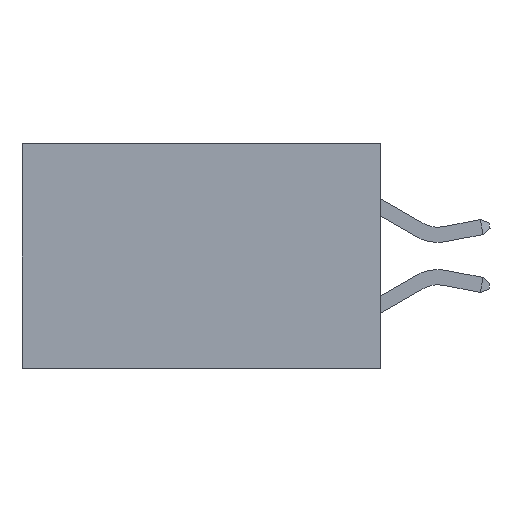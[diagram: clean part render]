
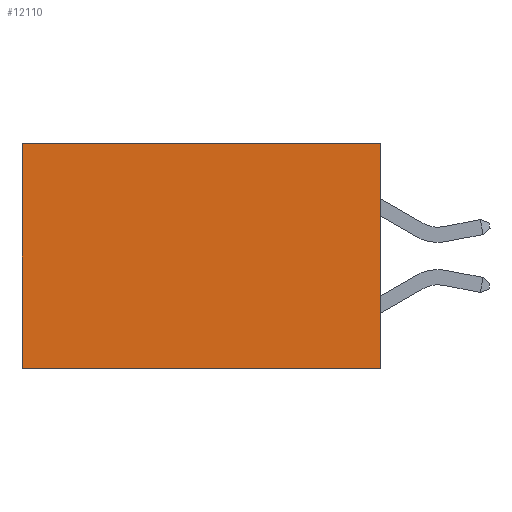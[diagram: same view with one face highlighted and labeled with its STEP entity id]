
A CAD part, left-side view. The second image highlights one B-rep face of the part: STEP entity #12110.
In plain terms, the highlighted planar face has unit normal (-1, 0, 0).
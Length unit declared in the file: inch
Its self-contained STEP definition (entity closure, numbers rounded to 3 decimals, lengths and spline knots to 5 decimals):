
#2889 = EDGE_CURVE ( 'NONE', #26231, #6369, #12886, .T. ) ;
#4138 = DIRECTION ( 'NONE',  ( 0., 0., -1. ) ) ;
#5319 = VECTOR ( 'NONE', #24436, 39.37008 ) ;
#6058 = CARTESIAN_POINT ( 'NONE',  ( 0.277, 0.59, -0.37 ) ) ;
#6369 = VERTEX_POINT ( 'NONE', #18548 ) ;
#8305 = PLANE ( 'NONE',  #18056 ) ;
#10510 = DIRECTION ( 'NONE',  ( 0., 0., -1. ) ) ;
#10622 = FACE_OUTER_BOUND ( 'NONE', #20371, .T. ) ;
#10805 = LINE ( 'NONE', #11871, #27906 ) ;
#10984 = CARTESIAN_POINT ( 'NONE',  ( 0.277, 0., -0.37 ) ) ;
#11871 = CARTESIAN_POINT ( 'NONE',  ( 0.277, 0., -0.37 ) ) ;
#12110 = ADVANCED_FACE ( 'NONE', ( #10622 ), #8305, .F. ) ;
#12886 = LINE ( 'NONE', #6058, #17498 ) ;
#12999 = EDGE_CURVE ( 'NONE', #14116, #25251, #23249, .T. ) ;
#13702 = ORIENTED_EDGE ( 'NONE', *, *, #18943, .T. ) ;
#14007 = LINE ( 'NONE', #21699, #25910 ) ;
#14116 = VERTEX_POINT ( 'NONE', #22072 ) ;
#14143 = DIRECTION ( 'NONE',  ( 0., 1., 0. ) ) ;
#15758 = EDGE_CURVE ( 'NONE', #25251, #6369, #10805, .T. ) ;
#17498 = VECTOR ( 'NONE', #4138, 39.37008 ) ;
#17536 = ORIENTED_EDGE ( 'NONE', *, *, #2889, .T. ) ;
#18056 = AXIS2_PLACEMENT_3D ( 'NONE', #28161, #23980, #10510 ) ;
#18548 = CARTESIAN_POINT ( 'NONE',  ( 0.277, 0.59, -0.37 ) ) ;
#18943 = EDGE_CURVE ( 'NONE', #14116, #26231, #14007, .T. ) ;
#19344 = ORIENTED_EDGE ( 'NONE', *, *, #15758, .F. ) ;
#20371 = EDGE_LOOP ( 'NONE', ( #17536, #19344, #27937, #13702 ) ) ;
#21305 = CARTESIAN_POINT ( 'NONE',  ( 0.277, 0., -0.37 ) ) ;
#21699 = CARTESIAN_POINT ( 'NONE',  ( 0.277, 0., 0. ) ) ;
#22072 = CARTESIAN_POINT ( 'NONE',  ( 0.277, 0., 0. ) ) ;
#23249 = LINE ( 'NONE', #10984, #5319 ) ;
#23926 = DIRECTION ( 'NONE',  ( 0., 1., 0. ) ) ;
#23980 = DIRECTION ( 'NONE',  ( 1., 0., 0. ) ) ;
#24436 = DIRECTION ( 'NONE',  ( 0., 0., -1. ) ) ;
#25251 = VERTEX_POINT ( 'NONE', #21305 ) ;
#25910 = VECTOR ( 'NONE', #23926, 39.37008 ) ;
#26231 = VERTEX_POINT ( 'NONE', #26665 ) ;
#26665 = CARTESIAN_POINT ( 'NONE',  ( 0.277, 0.59, 0. ) ) ;
#27906 = VECTOR ( 'NONE', #14143, 39.37008 ) ;
#27937 = ORIENTED_EDGE ( 'NONE', *, *, #12999, .F. ) ;
#28161 = CARTESIAN_POINT ( 'NONE',  ( 0.277, 0., -0.37 ) ) ;
